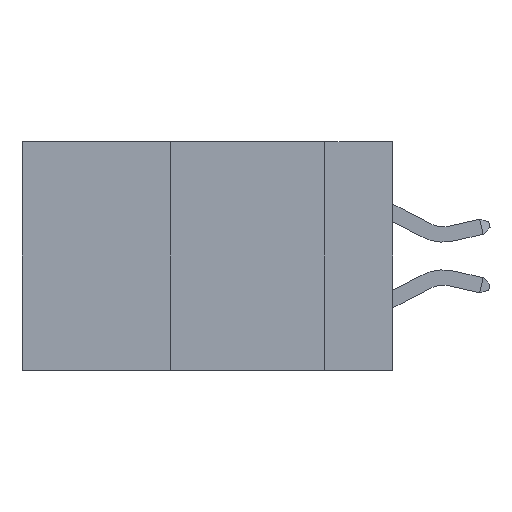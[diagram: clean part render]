
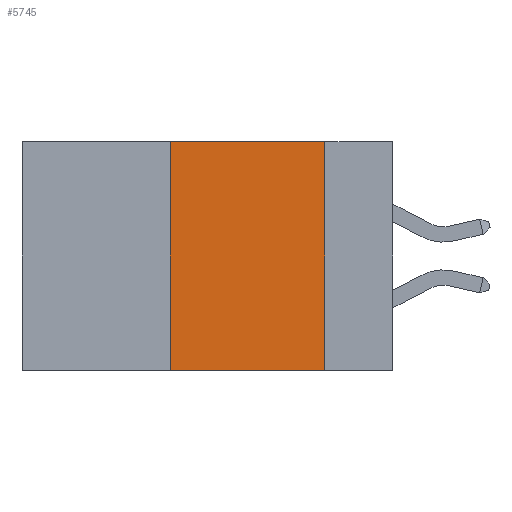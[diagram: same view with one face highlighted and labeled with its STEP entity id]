
A CAD part, left-side view. The second image highlights one B-rep face of the part: STEP entity #5745.
In plain terms, the highlighted planar face has unit normal (-1, 0, 0).
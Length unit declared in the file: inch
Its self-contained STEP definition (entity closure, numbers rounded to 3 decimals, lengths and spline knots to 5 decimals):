
#832 = VERTEX_POINT ( 'NONE', #21549 ) ;
#1174 = VERTEX_POINT ( 'NONE', #8016 ) ;
#2551 = PLANE ( 'NONE',  #14157 ) ;
#3596 = EDGE_CURVE ( 'NONE', #832, #1174, #14965, .T. ) ;
#4018 = VECTOR ( 'NONE', #5658, 39.37008 ) ;
#4531 = EDGE_CURVE ( 'NONE', #14747, #4619, #20162, .T. ) ;
#4619 = VERTEX_POINT ( 'NONE', #18540 ) ;
#5658 = DIRECTION ( 'NONE',  ( 0., -1., 0. ) ) ;
#5745 = ADVANCED_FACE ( 'NONE', ( #15114 ), #2551, .F. ) ;
#6556 = VECTOR ( 'NONE', #13081, 39.37008 ) ;
#6690 = VECTOR ( 'NONE', #29771, 39.37008 ) ;
#8016 = CARTESIAN_POINT ( 'NONE',  ( 0., 0.11, -0.37 ) ) ;
#8254 = LINE ( 'NONE', #22392, #4018 ) ;
#8916 = CARTESIAN_POINT ( 'NONE',  ( 0., 0.6, -0.37 ) ) ;
#9548 = LINE ( 'NONE', #8916, #30734 ) ;
#10342 = CARTESIAN_POINT ( 'NONE',  ( 0., 0.36, 0. ) ) ;
#13081 = DIRECTION ( 'NONE',  ( 0., 0., 1. ) ) ;
#14157 = AXIS2_PLACEMENT_3D ( 'NONE', #30074, #17524, #29597 ) ;
#14747 = VERTEX_POINT ( 'NONE', #15199 ) ;
#14965 = LINE ( 'NONE', #27350, #6690 ) ;
#15114 = FACE_OUTER_BOUND ( 'NONE', #21527, .T. ) ;
#15199 = CARTESIAN_POINT ( 'NONE',  ( 0., 0.36, -0.37 ) ) ;
#17524 = DIRECTION ( 'NONE',  ( 1., 0., 0. ) ) ;
#18540 = CARTESIAN_POINT ( 'NONE',  ( 0., 0.36, 0. ) ) ;
#20162 = LINE ( 'NONE', #10342, #6556 ) ;
#21527 = EDGE_LOOP ( 'NONE', ( #21657, #26671, #26667, #24868 ) ) ;
#21549 = CARTESIAN_POINT ( 'NONE',  ( 0., 0.11, 0. ) ) ;
#21657 = ORIENTED_EDGE ( 'NONE', *, *, #3596, .F. ) ;
#21837 = EDGE_CURVE ( 'NONE', #14747, #1174, #9548, .T. ) ;
#22392 = CARTESIAN_POINT ( 'NONE',  ( 0., 0.6, 0. ) ) ;
#24868 = ORIENTED_EDGE ( 'NONE', *, *, #21837, .T. ) ;
#26086 = EDGE_CURVE ( 'NONE', #4619, #832, #8254, .T. ) ;
#26667 = ORIENTED_EDGE ( 'NONE', *, *, #4531, .F. ) ;
#26671 = ORIENTED_EDGE ( 'NONE', *, *, #26086, .F. ) ;
#27350 = CARTESIAN_POINT ( 'NONE',  ( 0., 0.11, 0. ) ) ;
#28540 = DIRECTION ( 'NONE',  ( 0., -1., 0. ) ) ;
#29597 = DIRECTION ( 'NONE',  ( 0., 0., -1. ) ) ;
#29771 = DIRECTION ( 'NONE',  ( 0., 0., -1. ) ) ;
#30074 = CARTESIAN_POINT ( 'NONE',  ( 0., 0.6, 0. ) ) ;
#30734 = VECTOR ( 'NONE', #28540, 39.37008 ) ;
